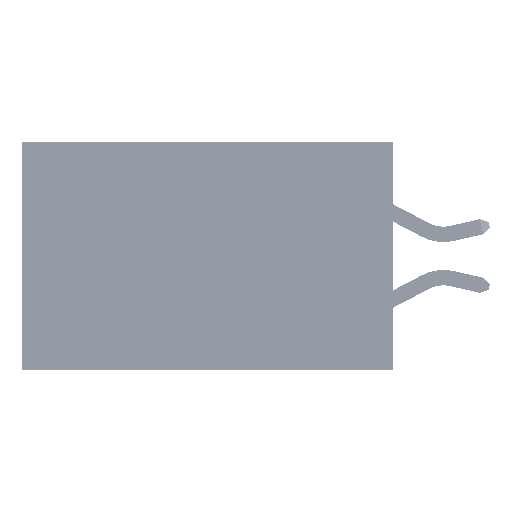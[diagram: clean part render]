
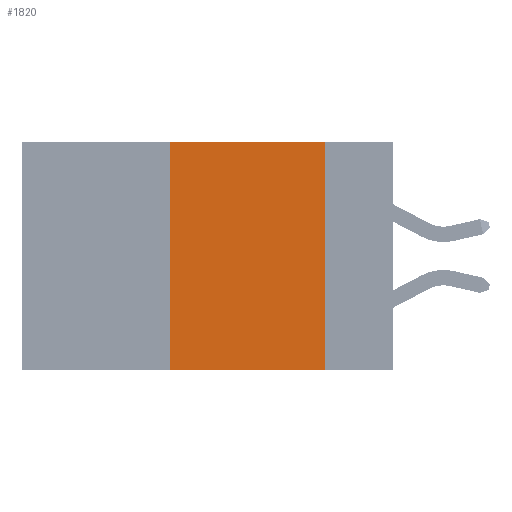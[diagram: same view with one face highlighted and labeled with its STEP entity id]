
A CAD part, left-side view. The second image highlights one B-rep face of the part: STEP entity #1820.
In plain terms, the highlighted planar face has unit normal (-1, 0, 0).
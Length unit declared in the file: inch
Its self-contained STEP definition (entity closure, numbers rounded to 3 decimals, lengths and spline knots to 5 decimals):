
#372 = CARTESIAN_POINT ( 'NONE',  ( 0., 0.11, -0.37 ) ) ;
#413 = VECTOR ( 'NONE', #18966, 39.37008 ) ;
#1500 = DIRECTION ( 'NONE',  ( 0., 0., -1. ) ) ;
#1820 = ADVANCED_FACE ( 'NONE', ( #44831 ), #33897, .F. ) ;
#11813 = CARTESIAN_POINT ( 'NONE',  ( 0., 0.6, 0. ) ) ;
#12030 = CARTESIAN_POINT ( 'NONE',  ( 0., 0.36, 0. ) ) ;
#12078 = ORIENTED_EDGE ( 'NONE', *, *, #24913, .F. ) ;
#12146 = DIRECTION ( 'NONE',  ( 0., -1., 0. ) ) ;
#12674 = LINE ( 'NONE', #30207, #413 ) ;
#12749 = EDGE_CURVE ( 'NONE', #21439, #37879, #12674, .T. ) ;
#12750 = VECTOR ( 'NONE', #12146, 39.37008 ) ;
#12980 = VECTOR ( 'NONE', #23614, 39.37008 ) ;
#16247 = CARTESIAN_POINT ( 'NONE',  ( 0., 0.11, 0. ) ) ;
#18029 = LINE ( 'NONE', #16247, #12980 ) ;
#18966 = DIRECTION ( 'NONE',  ( 0., -1., 0. ) ) ;
#19208 = CARTESIAN_POINT ( 'NONE',  ( 0., 0.6, -0.37 ) ) ;
#20069 = VECTOR ( 'NONE', #44293, 39.37008 ) ;
#20119 = EDGE_CURVE ( 'NONE', #37650, #21439, #41367, .T. ) ;
#21439 = VERTEX_POINT ( 'NONE', #22218 ) ;
#22218 = CARTESIAN_POINT ( 'NONE',  ( 0., 0.36, 0. ) ) ;
#23208 = EDGE_LOOP ( 'NONE', ( #12078, #40534, #23592, #38180 ) ) ;
#23464 = AXIS2_PLACEMENT_3D ( 'NONE', #11813, #29821, #1500 ) ;
#23592 = ORIENTED_EDGE ( 'NONE', *, *, #20119, .F. ) ;
#23614 = DIRECTION ( 'NONE',  ( 0., 0., -1. ) ) ;
#24913 = EDGE_CURVE ( 'NONE', #37879, #41814, #18029, .T. ) ;
#29821 = DIRECTION ( 'NONE',  ( 1., 0., 0. ) ) ;
#30207 = CARTESIAN_POINT ( 'NONE',  ( 0., 0.6, 0. ) ) ;
#30458 = CARTESIAN_POINT ( 'NONE',  ( 0., 0.36, -0.37 ) ) ;
#33897 = PLANE ( 'NONE',  #23464 ) ;
#34068 = LINE ( 'NONE', #19208, #12750 ) ;
#34730 = EDGE_CURVE ( 'NONE', #37650, #41814, #34068, .T. ) ;
#37650 = VERTEX_POINT ( 'NONE', #30458 ) ;
#37879 = VERTEX_POINT ( 'NONE', #39078 ) ;
#38180 = ORIENTED_EDGE ( 'NONE', *, *, #34730, .T. ) ;
#39078 = CARTESIAN_POINT ( 'NONE',  ( 0., 0.11, 0. ) ) ;
#40534 = ORIENTED_EDGE ( 'NONE', *, *, #12749, .F. ) ;
#41367 = LINE ( 'NONE', #12030, #20069 ) ;
#41814 = VERTEX_POINT ( 'NONE', #372 ) ;
#44293 = DIRECTION ( 'NONE',  ( 0., 0., 1. ) ) ;
#44831 = FACE_OUTER_BOUND ( 'NONE', #23208, .T. ) ;
